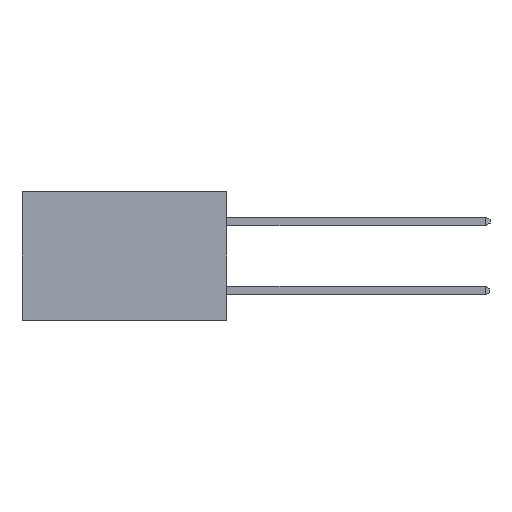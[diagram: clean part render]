
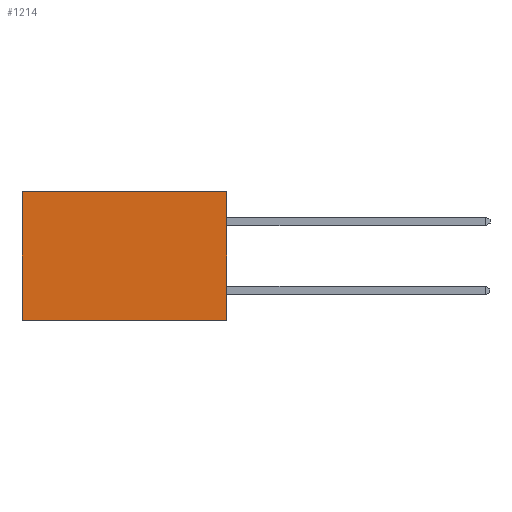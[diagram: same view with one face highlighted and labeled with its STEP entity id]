
A CAD part, left-side view. The second image highlights one B-rep face of the part: STEP entity #1214.
In plain terms, the highlighted planar face has unit normal (-1, 0, 0).
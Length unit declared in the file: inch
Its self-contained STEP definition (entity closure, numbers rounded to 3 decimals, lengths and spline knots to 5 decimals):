
#476 = CARTESIAN_POINT ( 'NONE',  ( 0.277, 0., -0.37 ) ) ;
#526 = VERTEX_POINT ( 'NONE', #1706 ) ;
#546 = VECTOR ( 'NONE', #5642, 39.37008 ) ;
#697 = ORIENTED_EDGE ( 'NONE', *, *, #3368, .F. ) ;
#739 = LINE ( 'NONE', #10874, #7888 ) ;
#849 = EDGE_LOOP ( 'NONE', ( #2193, #697, #10394, #1366 ) ) ;
#1214 = ADVANCED_FACE ( 'NONE', ( #12004 ), #7546, .F. ) ;
#1366 = ORIENTED_EDGE ( 'NONE', *, *, #6318, .T. ) ;
#1407 = CARTESIAN_POINT ( 'NONE',  ( 0.277, 0.59, 0. ) ) ;
#1472 = DIRECTION ( 'NONE',  ( 0., 1., 0. ) ) ;
#1706 = CARTESIAN_POINT ( 'NONE',  ( 0.277, 0.59, -0.37 ) ) ;
#1895 = CARTESIAN_POINT ( 'NONE',  ( 0.277, 0., -0.37 ) ) ;
#2193 = ORIENTED_EDGE ( 'NONE', *, *, #6598, .T. ) ;
#3368 = EDGE_CURVE ( 'NONE', #7830, #526, #10949, .T. ) ;
#3802 = LINE ( 'NONE', #8902, #8122 ) ;
#3845 = EDGE_CURVE ( 'NONE', #11755, #7830, #739, .T. ) ;
#4714 = CARTESIAN_POINT ( 'NONE',  ( 0.277, 0.59, -0.37 ) ) ;
#4768 = DIRECTION ( 'NONE',  ( 0., 0., -1. ) ) ;
#5028 = CARTESIAN_POINT ( 'NONE',  ( 0.277, 0., 0. ) ) ;
#5098 = VERTEX_POINT ( 'NONE', #1407 ) ;
#5626 = CARTESIAN_POINT ( 'NONE',  ( 0.277, 0., -0.37 ) ) ;
#5642 = DIRECTION ( 'NONE',  ( 0., 0., -1. ) ) ;
#5692 = DIRECTION ( 'NONE',  ( 0., 1., 0. ) ) ;
#5816 = LINE ( 'NONE', #4714, #546 ) ;
#5937 = AXIS2_PLACEMENT_3D ( 'NONE', #476, #9379, #11052 ) ;
#6318 = EDGE_CURVE ( 'NONE', #11755, #5098, #3802, .T. ) ;
#6598 = EDGE_CURVE ( 'NONE', #5098, #526, #5816, .T. ) ;
#7546 = PLANE ( 'NONE',  #5937 ) ;
#7830 = VERTEX_POINT ( 'NONE', #5626 ) ;
#7888 = VECTOR ( 'NONE', #4768, 39.37008 ) ;
#8122 = VECTOR ( 'NONE', #1472, 39.37008 ) ;
#8484 = VECTOR ( 'NONE', #5692, 39.37008 ) ;
#8902 = CARTESIAN_POINT ( 'NONE',  ( 0.277, 0., 0. ) ) ;
#9379 = DIRECTION ( 'NONE',  ( 1., 0., 0. ) ) ;
#10394 = ORIENTED_EDGE ( 'NONE', *, *, #3845, .F. ) ;
#10874 = CARTESIAN_POINT ( 'NONE',  ( 0.277, 0., -0.37 ) ) ;
#10949 = LINE ( 'NONE', #1895, #8484 ) ;
#11052 = DIRECTION ( 'NONE',  ( 0., 0., -1. ) ) ;
#11755 = VERTEX_POINT ( 'NONE', #5028 ) ;
#12004 = FACE_OUTER_BOUND ( 'NONE', #849, .T. ) ;
